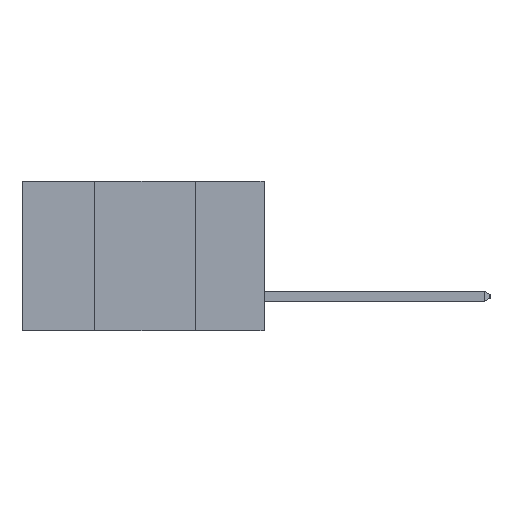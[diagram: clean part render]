
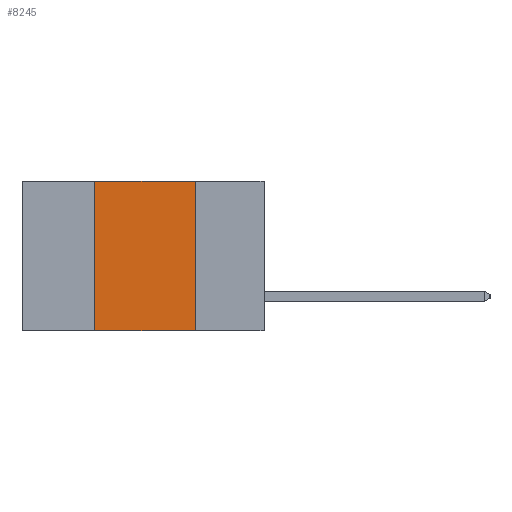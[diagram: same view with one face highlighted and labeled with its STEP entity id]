
A CAD part, left-side view. The second image highlights one B-rep face of the part: STEP entity #8245.
In plain terms, the highlighted planar face has unit normal (-1, 0, 0).
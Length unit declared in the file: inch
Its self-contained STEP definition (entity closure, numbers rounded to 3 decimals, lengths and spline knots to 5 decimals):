
#333 = VERTEX_POINT ( 'NONE', #3985 ) ;
#357 = PLANE ( 'NONE',  #5945 ) ;
#834 = VECTOR ( 'NONE', #5528, 39.37008 ) ;
#924 = VERTEX_POINT ( 'NONE', #6300 ) ;
#1024 = ORIENTED_EDGE ( 'NONE', *, *, #2109, .T. ) ;
#1047 = VECTOR ( 'NONE', #1740, 39.37008 ) ;
#1166 = DIRECTION ( 'NONE',  ( 0., 0., -1. ) ) ;
#1228 = DIRECTION ( 'NONE',  ( 0., -1., 0. ) ) ;
#1268 = ORIENTED_EDGE ( 'NONE', *, *, #4125, .F. ) ;
#1568 = CARTESIAN_POINT ( 'NONE',  ( 0., 0.6, 0. ) ) ;
#1740 = DIRECTION ( 'NONE',  ( 0., -1., 0. ) ) ;
#2004 = LINE ( 'NONE', #3752, #9816 ) ;
#2109 = EDGE_CURVE ( 'NONE', #4058, #3002, #2004, .T. ) ;
#2306 = EDGE_CURVE ( 'NONE', #4058, #333, #4244, .T. ) ;
#2719 = LINE ( 'NONE', #5535, #834 ) ;
#3002 = VERTEX_POINT ( 'NONE', #8823 ) ;
#3166 = ORIENTED_EDGE ( 'NONE', *, *, #2306, .F. ) ;
#3408 = DIRECTION ( 'NONE',  ( 0., 0., 1. ) ) ;
#3432 = EDGE_LOOP ( 'NONE', ( #1268, #5237, #3166, #1024 ) ) ;
#3752 = CARTESIAN_POINT ( 'NONE',  ( 0., 0.6, -0.37 ) ) ;
#3985 = CARTESIAN_POINT ( 'NONE',  ( 0., 0.42, 0. ) ) ;
#4058 = VERTEX_POINT ( 'NONE', #4715 ) ;
#4125 = EDGE_CURVE ( 'NONE', #924, #3002, #2719, .T. ) ;
#4244 = LINE ( 'NONE', #5296, #9915 ) ;
#4715 = CARTESIAN_POINT ( 'NONE',  ( 0., 0.42, -0.37 ) ) ;
#5115 = CARTESIAN_POINT ( 'NONE',  ( 0., 0.6, 0. ) ) ;
#5237 = ORIENTED_EDGE ( 'NONE', *, *, #5888, .F. ) ;
#5296 = CARTESIAN_POINT ( 'NONE',  ( 0., 0.42, -0.37 ) ) ;
#5528 = DIRECTION ( 'NONE',  ( 0., 0., -1. ) ) ;
#5535 = CARTESIAN_POINT ( 'NONE',  ( 0., 0.17, -0.37 ) ) ;
#5705 = FACE_OUTER_BOUND ( 'NONE', #3432, .T. ) ;
#5888 = EDGE_CURVE ( 'NONE', #333, #924, #7024, .T. ) ;
#5909 = DIRECTION ( 'NONE',  ( 1., 0., 0. ) ) ;
#5945 = AXIS2_PLACEMENT_3D ( 'NONE', #5115, #5909, #1166 ) ;
#6300 = CARTESIAN_POINT ( 'NONE',  ( 0., 0.17, 0. ) ) ;
#7024 = LINE ( 'NONE', #1568, #1047 ) ;
#8245 = ADVANCED_FACE ( 'NONE', ( #5705 ), #357, .F. ) ;
#8823 = CARTESIAN_POINT ( 'NONE',  ( 0., 0.17, -0.37 ) ) ;
#9816 = VECTOR ( 'NONE', #1228, 39.37008 ) ;
#9915 = VECTOR ( 'NONE', #3408, 39.37008 ) ;
